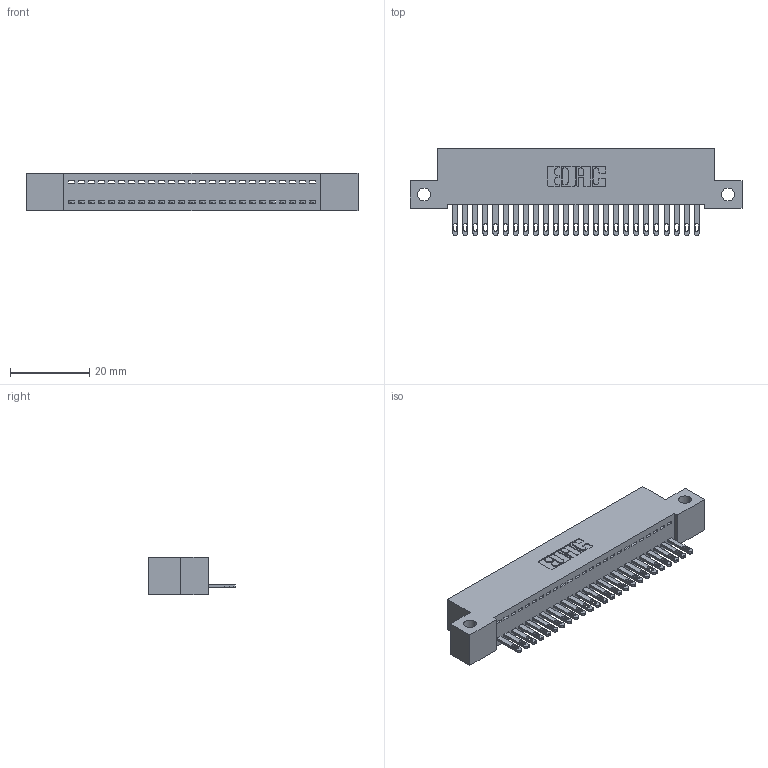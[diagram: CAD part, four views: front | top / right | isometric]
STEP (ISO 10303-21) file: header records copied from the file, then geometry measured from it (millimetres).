
FILE_DESCRIPTION (( 'STEP AP203' ), '1' );
FILE_NAME ('892-025-500-112.STEP', '2020-09-21T14:33:30', ( '' ), ( '' ), 'SwSTEP 2.0', 'SolidWorks 2020', '' );
FILE_SCHEMA (( 'CONFIG_CONTROL_DESIGN' ));
Length unit declared in the file: inch
Products named in the file (3): 892-025-500-112; 842 Part_Side Mount; 345-292-001_345-293-100
Assembly tree (26 placements, depth 2):
  892-025-500-112
    842 Part_Side Mount
    345-292-001_345-293-100  x25
Bounding box: 83.82 x 21.85 x 9.4 mm (x, y, z)
Volume: 7228.3 mm3; surface area: 10183.1 mm2
Topology: 26 solids, 26 shells, 1460 faces, 4499 edges, 2998 vertices
Faces by surface type: plane 966, cylinder 494
Entity records: 17283 total; most frequent: CARTESIAN_POINT 2989, ORIENTED_EDGE 2950, DIRECTION 2557, EDGE_CURVE 1475, VECTOR 1343, LINE 1343, VERTEX_POINT 982, AXIS2_PLACEMENT_3D 607
